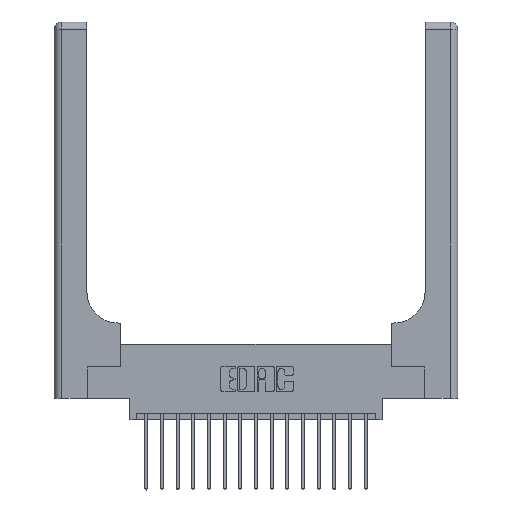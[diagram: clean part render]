
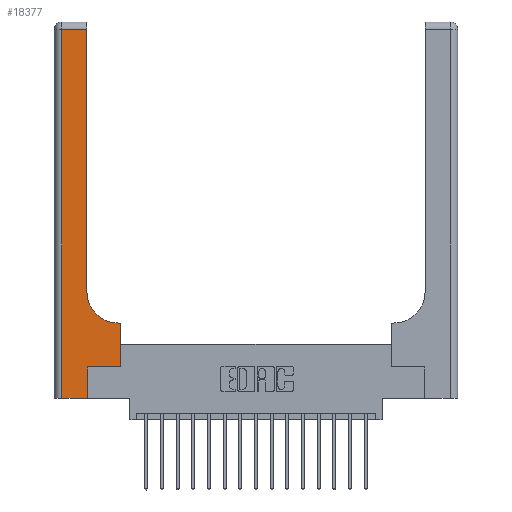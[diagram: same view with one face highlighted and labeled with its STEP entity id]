
A CAD part, top view. The second image highlights one B-rep face of the part: STEP entity #18377.
In plain terms, the highlighted planar face has unit normal (0, 0, 1).
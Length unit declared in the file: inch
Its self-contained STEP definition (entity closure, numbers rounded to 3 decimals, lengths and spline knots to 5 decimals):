
#662 = CARTESIAN_POINT ( 'NONE',  ( 0.528, 0.25, 0.37 ) ) ;
#750 = DIRECTION ( 'NONE',  ( 0., -1., 0. ) ) ;
#848 = VECTOR ( 'NONE', #750, 39.37008 ) ;
#1015 = EDGE_LOOP ( 'NONE', ( #7315, #12531, #3255, #14813, #11394, #17099, #10271, #14131, #4860 ) ) ;
#1054 = CARTESIAN_POINT ( 'NONE',  ( 0., 0., 0.37 ) ) ;
#1074 = CARTESIAN_POINT ( 'NONE',  ( 0.51, 0.85, 0.37 ) ) ;
#1123 = DIRECTION ( 'NONE',  ( 1., 0., 0. ) ) ;
#1171 = EDGE_CURVE ( 'NONE', #15775, #18390, #12400, .T. ) ;
#1249 = CARTESIAN_POINT ( 'NONE',  ( 0.06, 0., 0.37 ) ) ;
#1522 = CIRCLE ( 'NONE', #6061, 0.25 ) ;
#1680 = CARTESIAN_POINT ( 'NONE',  ( 0.265, 0., 0.37 ) ) ;
#1716 = LINE ( 'NONE', #3956, #8961 ) ;
#1893 = VECTOR ( 'NONE', #15684, 39.37008 ) ;
#2257 = VERTEX_POINT ( 'NONE', #16222 ) ;
#2387 = CARTESIAN_POINT ( 'NONE',  ( 0.26, 2.94, 0.37 ) ) ;
#2522 = DIRECTION ( 'NONE',  ( 1., 0., 0. ) ) ;
#2564 = CARTESIAN_POINT ( 'NONE',  ( 0.06, 2.94, 0.37 ) ) ;
#2708 = DIRECTION ( 'NONE',  ( -1., 0., 0. ) ) ;
#2812 = VECTOR ( 'NONE', #1123, 39.37008 ) ;
#3216 = EDGE_CURVE ( 'NONE', #18390, #7193, #18221, .T. ) ;
#3255 = ORIENTED_EDGE ( 'NONE', *, *, #1171, .T. ) ;
#3275 = EDGE_CURVE ( 'NONE', #16217, #4413, #13910, .T. ) ;
#3956 = CARTESIAN_POINT ( 'NONE',  ( 0.528, 0.25, 0.37 ) ) ;
#4005 = VECTOR ( 'NONE', #13280, 39.37008 ) ;
#4413 = VERTEX_POINT ( 'NONE', #2387 ) ;
#4483 = VERTEX_POINT ( 'NONE', #14099 ) ;
#4860 = ORIENTED_EDGE ( 'NONE', *, *, #13550, .T. ) ;
#5489 = DIRECTION ( 'NONE',  ( -1., 0., 0. ) ) ;
#6061 = AXIS2_PLACEMENT_3D ( 'NONE', #1074, #11189, #2522 ) ;
#6133 = CARTESIAN_POINT ( 'NONE',  ( 0.26, 0.6, 0.37 ) ) ;
#6608 = LINE ( 'NONE', #6133, #12289 ) ;
#6883 = DIRECTION ( 'NONE',  ( 1., 0., 0. ) ) ;
#7193 = VERTEX_POINT ( 'NONE', #8414 ) ;
#7315 = ORIENTED_EDGE ( 'NONE', *, *, #3275, .T. ) ;
#7762 = EDGE_CURVE ( 'NONE', #2257, #12766, #17062, .T. ) ;
#7954 = EDGE_CURVE ( 'NONE', #11002, #4483, #6608, .T. ) ;
#8414 = CARTESIAN_POINT ( 'NONE',  ( 0.265, 0., 0.37 ) ) ;
#8440 = PLANE ( 'NONE',  #12707 ) ;
#8918 = EDGE_CURVE ( 'NONE', #4413, #15775, #14745, .T. ) ;
#8961 = VECTOR ( 'NONE', #15554, 39.37008 ) ;
#9262 = CARTESIAN_POINT ( 'NONE',  ( 0.528, 0.6, 0.37 ) ) ;
#10271 = ORIENTED_EDGE ( 'NONE', *, *, #14225, .T. ) ;
#10422 = VECTOR ( 'NONE', #5489, 39.37008 ) ;
#11002 = VERTEX_POINT ( 'NONE', #9262 ) ;
#11189 = DIRECTION ( 'NONE',  ( 0., 0., -1. ) ) ;
#11361 = DIRECTION ( 'NONE',  ( 0., 0., -1. ) ) ;
#11394 = ORIENTED_EDGE ( 'NONE', *, *, #18618, .T. ) ;
#11479 = FACE_OUTER_BOUND ( 'NONE', #1015, .T. ) ;
#11695 = LINE ( 'NONE', #1680, #4005 ) ;
#12175 = CARTESIAN_POINT ( 'NONE',  ( 0.26, 0.85, 0.37 ) ) ;
#12289 = VECTOR ( 'NONE', #16278, 39.37008 ) ;
#12400 = LINE ( 'NONE', #18093, #848 ) ;
#12531 = ORIENTED_EDGE ( 'NONE', *, *, #8918, .T. ) ;
#12707 = AXIS2_PLACEMENT_3D ( 'NONE', #18605, #11361, #2708 ) ;
#12766 = VERTEX_POINT ( 'NONE', #662 ) ;
#13205 = VECTOR ( 'NONE', #6883, 39.37008 ) ;
#13280 = DIRECTION ( 'NONE',  ( 0., 1., 0. ) ) ;
#13550 = EDGE_CURVE ( 'NONE', #4483, #16217, #1522, .T. ) ;
#13910 = LINE ( 'NONE', #18596, #1893 ) ;
#14099 = CARTESIAN_POINT ( 'NONE',  ( 0.51, 0.6, 0.37 ) ) ;
#14121 = CARTESIAN_POINT ( 'NONE',  ( 0.265, 0.25, 0.37 ) ) ;
#14131 = ORIENTED_EDGE ( 'NONE', *, *, #7954, .T. ) ;
#14225 = EDGE_CURVE ( 'NONE', #12766, #11002, #1716, .T. ) ;
#14745 = LINE ( 'NONE', #17097, #10422 ) ;
#14813 = ORIENTED_EDGE ( 'NONE', *, *, #3216, .T. ) ;
#15554 = DIRECTION ( 'NONE',  ( 0., 1., 0. ) ) ;
#15684 = DIRECTION ( 'NONE',  ( 0., 1., 0. ) ) ;
#15775 = VERTEX_POINT ( 'NONE', #2564 ) ;
#16217 = VERTEX_POINT ( 'NONE', #12175 ) ;
#16222 = CARTESIAN_POINT ( 'NONE',  ( 0.265, 0.25, 0.37 ) ) ;
#16278 = DIRECTION ( 'NONE',  ( -1., 0., 0. ) ) ;
#17062 = LINE ( 'NONE', #14121, #13205 ) ;
#17097 = CARTESIAN_POINT ( 'NONE',  ( 0., 2.94, 0.37 ) ) ;
#17099 = ORIENTED_EDGE ( 'NONE', *, *, #7762, .T. ) ;
#18093 = CARTESIAN_POINT ( 'NONE',  ( 0.06, 3., 0.37 ) ) ;
#18221 = LINE ( 'NONE', #1054, #2812 ) ;
#18377 = ADVANCED_FACE ( 'NONE', ( #11479 ), #8440, .F. ) ;
#18390 = VERTEX_POINT ( 'NONE', #1249 ) ;
#18596 = CARTESIAN_POINT ( 'NONE',  ( 0.26, 3., 0.37 ) ) ;
#18605 = CARTESIAN_POINT ( 'NONE',  ( 0., 3., 0.37 ) ) ;
#18618 = EDGE_CURVE ( 'NONE', #7193, #2257, #11695, .T. ) ;
